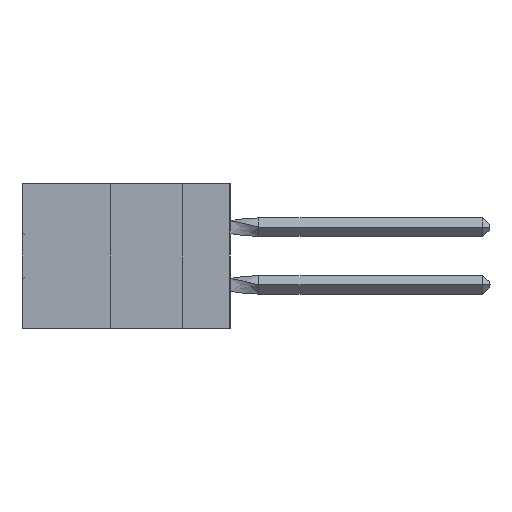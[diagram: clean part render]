
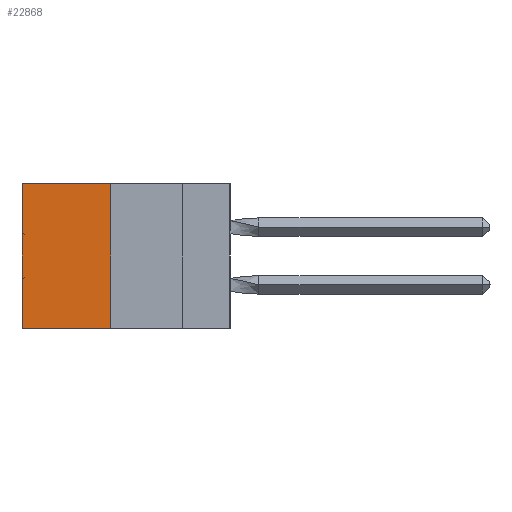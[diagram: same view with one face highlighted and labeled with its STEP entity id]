
A CAD part, left-side view. The second image highlights one B-rep face of the part: STEP entity #22868.
In plain terms, the highlighted planar face has unit normal (-1, 0, 0).
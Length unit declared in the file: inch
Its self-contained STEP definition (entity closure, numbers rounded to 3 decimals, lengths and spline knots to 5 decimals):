
#5347 = CARTESIAN_POINT ( 'NONE',  ( 0.305, 0.413, -0.5 ) ) ;
#5533 = VERTEX_POINT ( 'NONE', #5347 ) ;
#9334 = AXIS2_PLACEMENT_3D ( 'NONE', #37729, #20056, #37360 ) ;
#11066 = LINE ( 'NONE', #55670, #52919 ) ;
#11852 = LINE ( 'NONE', #37595, #55076 ) ;
#17711 = EDGE_CURVE ( 'NONE', #5533, #53354, #11852, .T. ) ;
#18926 = LINE ( 'NONE', #25089, #41550 ) ;
#19652 = CARTESIAN_POINT ( 'NONE',  ( 0.305, 0.72, -0.5 ) ) ;
#19857 = PLANE ( 'NONE',  #9334 ) ;
#20056 = DIRECTION ( 'NONE',  ( 1., 0., 0. ) ) ;
#20487 = DIRECTION ( 'NONE',  ( 0., 1., 0. ) ) ;
#21490 = EDGE_CURVE ( 'NONE', #39974, #53354, #50494, .T. ) ;
#22868 = ADVANCED_FACE ( 'NONE', ( #28441 ), #19857, .F. ) ;
#25089 = CARTESIAN_POINT ( 'NONE',  ( 0.305, 0.413, -0.5 ) ) ;
#27391 = CARTESIAN_POINT ( 'NONE',  ( 0.305, 0.413, 0. ) ) ;
#28111 = DIRECTION ( 'NONE',  ( 0., 0., -1. ) ) ;
#28441 = FACE_OUTER_BOUND ( 'NONE', #32063, .T. ) ;
#29803 = ORIENTED_EDGE ( 'NONE', *, *, #17711, .F. ) ;
#32035 = VECTOR ( 'NONE', #28111, 39.37008 ) ;
#32063 = EDGE_LOOP ( 'NONE', ( #39644, #29803, #38030, #54855 ) ) ;
#32219 = EDGE_CURVE ( 'NONE', #34654, #5533, #18926, .T. ) ;
#32767 = CARTESIAN_POINT ( 'NONE',  ( 0.305, 0.72, 0. ) ) ;
#34654 = VERTEX_POINT ( 'NONE', #27391 ) ;
#35002 = EDGE_CURVE ( 'NONE', #34654, #39974, #11066, .T. ) ;
#37360 = DIRECTION ( 'NONE',  ( 0., 0., -1. ) ) ;
#37595 = CARTESIAN_POINT ( 'NONE',  ( 0.305, 0.413, -0.5 ) ) ;
#37729 = CARTESIAN_POINT ( 'NONE',  ( 0.305, 0.413, -0.5 ) ) ;
#38030 = ORIENTED_EDGE ( 'NONE', *, *, #32219, .F. ) ;
#39644 = ORIENTED_EDGE ( 'NONE', *, *, #21490, .T. ) ;
#39974 = VERTEX_POINT ( 'NONE', #32767 ) ;
#41550 = VECTOR ( 'NONE', #43127, 39.37008 ) ;
#43127 = DIRECTION ( 'NONE',  ( 0., 0., -1. ) ) ;
#50494 = LINE ( 'NONE', #19652, #32035 ) ;
#52054 = DIRECTION ( 'NONE',  ( 0., 1., 0. ) ) ;
#52919 = VECTOR ( 'NONE', #52054, 39.37008 ) ;
#53354 = VERTEX_POINT ( 'NONE', #53690 ) ;
#53690 = CARTESIAN_POINT ( 'NONE',  ( 0.305, 0.72, -0.5 ) ) ;
#54855 = ORIENTED_EDGE ( 'NONE', *, *, #35002, .T. ) ;
#55076 = VECTOR ( 'NONE', #20487, 39.37008 ) ;
#55670 = CARTESIAN_POINT ( 'NONE',  ( 0.305, 0.413, 0. ) ) ;
